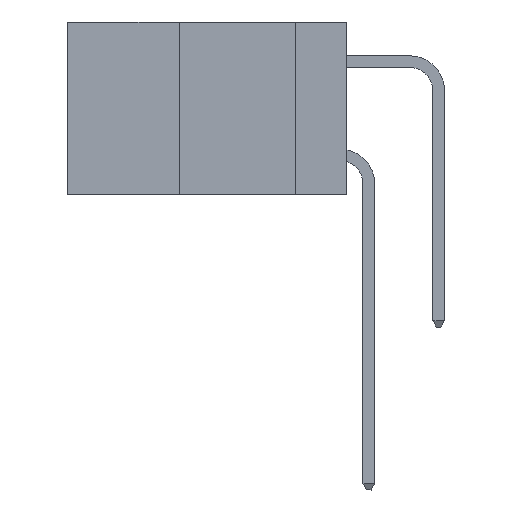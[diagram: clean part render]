
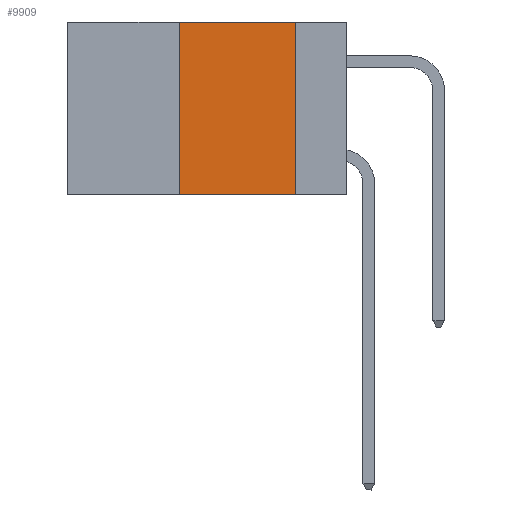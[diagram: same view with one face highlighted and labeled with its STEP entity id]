
A CAD part, left-side view. The second image highlights one B-rep face of the part: STEP entity #9909.
In plain terms, the highlighted planar face has unit normal (-1, 0, 0).
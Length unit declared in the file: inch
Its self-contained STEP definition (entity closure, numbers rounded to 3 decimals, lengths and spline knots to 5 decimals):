
#287 = AXIS2_PLACEMENT_3D ( 'NONE', #6768, #14744, #12910 ) ;
#1159 = VERTEX_POINT ( 'NONE', #19023 ) ;
#1559 = VECTOR ( 'NONE', #6473, 39.37008 ) ;
#2891 = DIRECTION ( 'NONE',  ( 0., -1., 0. ) ) ;
#2920 = VERTEX_POINT ( 'NONE', #14299 ) ;
#3096 = VERTEX_POINT ( 'NONE', #5475 ) ;
#3270 = CARTESIAN_POINT ( 'NONE',  ( 0., 0.11, 0. ) ) ;
#3883 = FACE_OUTER_BOUND ( 'NONE', #8810, .T. ) ;
#5475 = CARTESIAN_POINT ( 'NONE',  ( 0., 0.36, -0.37 ) ) ;
#5768 = EDGE_CURVE ( 'NONE', #1159, #2920, #7049, .T. ) ;
#6473 = DIRECTION ( 'NONE',  ( 0., 0., 1. ) ) ;
#6694 = CARTESIAN_POINT ( 'NONE',  ( 0., 0.11, -0.37 ) ) ;
#6768 = CARTESIAN_POINT ( 'NONE',  ( 0., 0.6, 0. ) ) ;
#7049 = LINE ( 'NONE', #7353, #9052 ) ;
#7237 = VECTOR ( 'NONE', #2891, 39.37008 ) ;
#7353 = CARTESIAN_POINT ( 'NONE',  ( 0., 0.6, 0. ) ) ;
#8503 = LINE ( 'NONE', #17613, #1559 ) ;
#8644 = EDGE_CURVE ( 'NONE', #3096, #1159, #8503, .T. ) ;
#8810 = EDGE_LOOP ( 'NONE', ( #15269, #19582, #14081, #16974 ) ) ;
#9052 = VECTOR ( 'NONE', #16663, 39.37008 ) ;
#9521 = DIRECTION ( 'NONE',  ( 0., 0., -1. ) ) ;
#9909 = ADVANCED_FACE ( 'NONE', ( #3883 ), #14448, .F. ) ;
#10683 = CARTESIAN_POINT ( 'NONE',  ( 0., 0.6, -0.37 ) ) ;
#12896 = VERTEX_POINT ( 'NONE', #6694 ) ;
#12910 = DIRECTION ( 'NONE',  ( 0., 0., -1. ) ) ;
#14081 = ORIENTED_EDGE ( 'NONE', *, *, #8644, .F. ) ;
#14132 = LINE ( 'NONE', #3270, #16446 ) ;
#14299 = CARTESIAN_POINT ( 'NONE',  ( 0., 0.11, 0. ) ) ;
#14448 = PLANE ( 'NONE',  #287 ) ;
#14449 = EDGE_CURVE ( 'NONE', #3096, #12896, #17013, .T. ) ;
#14744 = DIRECTION ( 'NONE',  ( 1., 0., 0. ) ) ;
#15269 = ORIENTED_EDGE ( 'NONE', *, *, #16086, .F. ) ;
#16086 = EDGE_CURVE ( 'NONE', #2920, #12896, #14132, .T. ) ;
#16446 = VECTOR ( 'NONE', #9521, 39.37008 ) ;
#16663 = DIRECTION ( 'NONE',  ( 0., -1., 0. ) ) ;
#16974 = ORIENTED_EDGE ( 'NONE', *, *, #14449, .T. ) ;
#17013 = LINE ( 'NONE', #10683, #7237 ) ;
#17613 = CARTESIAN_POINT ( 'NONE',  ( 0., 0.36, 0. ) ) ;
#19023 = CARTESIAN_POINT ( 'NONE',  ( 0., 0.36, 0. ) ) ;
#19582 = ORIENTED_EDGE ( 'NONE', *, *, #5768, .F. ) ;
